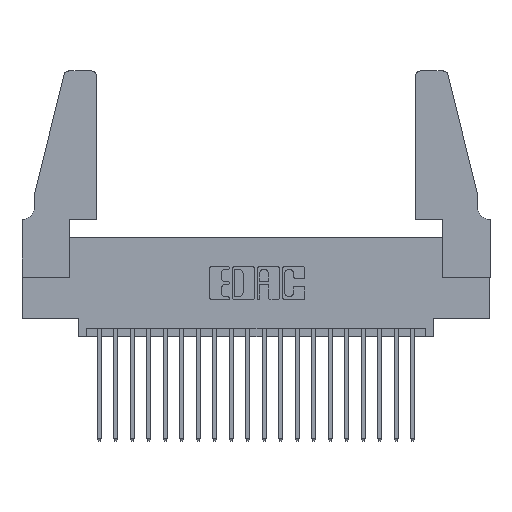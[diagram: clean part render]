
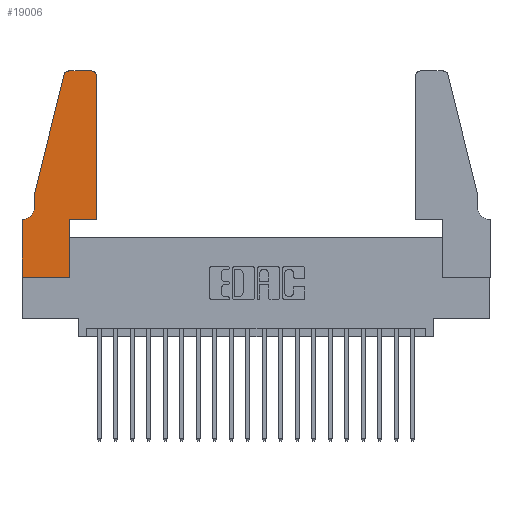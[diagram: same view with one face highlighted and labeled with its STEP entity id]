
A CAD part, top view. The second image highlights one B-rep face of the part: STEP entity #19006.
In plain terms, the highlighted planar face has unit normal (0, 0, 1).
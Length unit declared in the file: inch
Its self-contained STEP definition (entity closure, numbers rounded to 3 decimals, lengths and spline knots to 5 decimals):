
#118 = ORIENTED_EDGE ( 'NONE', *, *, #17093, .T. ) ;
#174 = LINE ( 'NONE', #9430, #17490 ) ;
#403 = CARTESIAN_POINT ( 'NONE',  ( 0.2865, 0., 0.37 ) ) ;
#721 = VERTEX_POINT ( 'NONE', #2761 ) ;
#1206 = ORIENTED_EDGE ( 'NONE', *, *, #18844, .T. ) ;
#1313 = VERTEX_POINT ( 'NONE', #9308 ) ;
#1337 = CARTESIAN_POINT ( 'NONE',  ( 0.0755, 0.42, 0.37 ) ) ;
#1368 = LINE ( 'NONE', #7653, #4801 ) ;
#1587 = EDGE_CURVE ( 'NONE', #721, #8507, #1368, .T. ) ;
#1672 = EDGE_CURVE ( 'NONE', #16099, #2057, #3743, .T. ) ;
#2003 = CARTESIAN_POINT ( 'NONE',  ( 0.0055, 0.35, 0.37 ) ) ;
#2057 = VERTEX_POINT ( 'NONE', #11794 ) ;
#2196 = DIRECTION ( 'NONE',  ( -1., 0., 0. ) ) ;
#2416 = LINE ( 'NONE', #7904, #14903 ) ;
#2524 = ORIENTED_EDGE ( 'NONE', *, *, #1587, .T. ) ;
#2761 = CARTESIAN_POINT ( 'NONE',  ( 0.0755, 0.5, 0.37 ) ) ;
#2979 = DIRECTION ( 'NONE',  ( 1., 0., 0. ) ) ;
#2988 = ORIENTED_EDGE ( 'NONE', *, *, #8471, .T. ) ;
#3020 = AXIS2_PLACEMENT_3D ( 'NONE', #13371, #3627, #14956 ) ;
#3223 = VECTOR ( 'NONE', #11730, 39.37008 ) ;
#3501 = VERTEX_POINT ( 'NONE', #4126 ) ;
#3627 = DIRECTION ( 'NONE',  ( 0., 0., -1. ) ) ;
#3743 = LINE ( 'NONE', #11330, #3223 ) ;
#3797 = CARTESIAN_POINT ( 'NONE',  ( 0., 0.35, 0.37 ) ) ;
#3916 = CARTESIAN_POINT ( 'NONE',  ( 0.2605, 1.25, 0.37 ) ) ;
#4104 = VERTEX_POINT ( 'NONE', #10342 ) ;
#4126 = CARTESIAN_POINT ( 'NONE',  ( 0.284, 1.25, 0.37 ) ) ;
#4167 = CIRCLE ( 'NONE', #3020, 0.07 ) ;
#4284 = CARTESIAN_POINT ( 'NONE',  ( 0., 0., 0.37 ) ) ;
#4291 = DIRECTION ( 'NONE',  ( 0., 0., 1. ) ) ;
#4454 = ORIENTED_EDGE ( 'NONE', *, *, #9202, .T. ) ;
#4553 = CARTESIAN_POINT ( 'NONE',  ( 0.0755, 0.35, 0.37 ) ) ;
#4801 = VECTOR ( 'NONE', #13757, 39.37008 ) ;
#5517 = EDGE_CURVE ( 'NONE', #1313, #721, #19964, .T. ) ;
#5523 = VECTOR ( 'NONE', #17160, 39.37008 ) ;
#6093 = CARTESIAN_POINT ( 'NONE',  ( 0.284, 1.22, 0.37 ) ) ;
#6197 = ORIENTED_EDGE ( 'NONE', *, *, #1672, .T. ) ;
#6291 = ORIENTED_EDGE ( 'NONE', *, *, #14960, .T. ) ;
#6374 = CARTESIAN_POINT ( 'NONE',  ( 0., 0.35, 0.37 ) ) ;
#7531 = VECTOR ( 'NONE', #17345, 39.37008 ) ;
#7577 = ORIENTED_EDGE ( 'NONE', *, *, #10851, .T. ) ;
#7653 = CARTESIAN_POINT ( 'NONE',  ( 0.0755, 0.5, 0.37 ) ) ;
#7717 = DIRECTION ( 'NONE',  ( 0., 1., 0. ) ) ;
#7752 = DIRECTION ( 'NONE',  ( 1., 0., 0. ) ) ;
#7781 = CIRCLE ( 'NONE', #16152, 0.03 ) ;
#7857 = CARTESIAN_POINT ( 'NONE',  ( 0.4505, 0.35, 0.37 ) ) ;
#7876 = LINE ( 'NONE', #3916, #11656 ) ;
#7904 = CARTESIAN_POINT ( 'NONE',  ( 0., 0., 0.37 ) ) ;
#8020 = DIRECTION ( 'NONE',  ( 1., 0., 0. ) ) ;
#8045 = LINE ( 'NONE', #4553, #7531 ) ;
#8194 = ORIENTED_EDGE ( 'NONE', *, *, #17088, .T. ) ;
#8471 = EDGE_CURVE ( 'NONE', #10983, #10226, #2416, .T. ) ;
#8507 = VERTEX_POINT ( 'NONE', #1337 ) ;
#8801 = CARTESIAN_POINT ( 'NONE',  ( 0., 0., 0.37 ) ) ;
#8849 = EDGE_CURVE ( 'NONE', #11678, #3501, #7876, .T. ) ;
#8924 = CARTESIAN_POINT ( 'NONE',  ( 0.4205, 1.25, 0.37 ) ) ;
#9202 = EDGE_CURVE ( 'NONE', #15530, #10983, #9892, .T. ) ;
#9308 = CARTESIAN_POINT ( 'NONE',  ( 0.25487, 1.22718, 0.37 ) ) ;
#9430 = CARTESIAN_POINT ( 'NONE',  ( 0.2865, 0.35, 0.37 ) ) ;
#9485 = DIRECTION ( 'NONE',  ( 1., 0., 0. ) ) ;
#9892 = LINE ( 'NONE', #4284, #5523 ) ;
#10226 = VERTEX_POINT ( 'NONE', #403 ) ;
#10281 = ORIENTED_EDGE ( 'NONE', *, *, #8849, .T. ) ;
#10342 = CARTESIAN_POINT ( 'NONE',  ( 0.2865, 0.35, 0.37 ) ) ;
#10851 = EDGE_CURVE ( 'NONE', #8507, #15477, #4167, .T. ) ;
#10983 = VERTEX_POINT ( 'NONE', #8801 ) ;
#11314 = AXIS2_PLACEMENT_3D ( 'NONE', #6093, #17316, #7752 ) ;
#11330 = CARTESIAN_POINT ( 'NONE',  ( 0.4505, 0.35, 0.37 ) ) ;
#11512 = AXIS2_PLACEMENT_3D ( 'NONE', #6374, #17588, #8020 ) ;
#11543 = EDGE_LOOP ( 'NONE', ( #10281, #6291, #12653, #2524, #7577, #8194, #4454, #2988, #20379, #118, #6197, #1206 ) ) ;
#11554 = VECTOR ( 'NONE', #16802, 39.37008 ) ;
#11656 = VECTOR ( 'NONE', #2196, 39.37008 ) ;
#11678 = VERTEX_POINT ( 'NONE', #8924 ) ;
#11730 = DIRECTION ( 'NONE',  ( 0., 1., 0. ) ) ;
#11794 = CARTESIAN_POINT ( 'NONE',  ( 0.4505, 1.22, 0.37 ) ) ;
#11829 = CARTESIAN_POINT ( 'NONE',  ( 0.4505, 0.35, 0.37 ) ) ;
#11891 = EDGE_CURVE ( 'NONE', #10226, #4104, #174, .T. ) ;
#12023 = CARTESIAN_POINT ( 'NONE',  ( 0.0755, 0.5, 0.37 ) ) ;
#12653 = ORIENTED_EDGE ( 'NONE', *, *, #5517, .T. ) ;
#12817 = PLANE ( 'NONE',  #11512 ) ;
#13371 = CARTESIAN_POINT ( 'NONE',  ( 0.0055, 0.42, 0.37 ) ) ;
#13757 = DIRECTION ( 'NONE',  ( 0., -1., 0. ) ) ;
#13994 = CARTESIAN_POINT ( 'NONE',  ( 0.4205, 1.22, 0.37 ) ) ;
#14903 = VECTOR ( 'NONE', #2979, 39.37008 ) ;
#14956 = DIRECTION ( 'NONE',  ( -1., 0., 0. ) ) ;
#14960 = EDGE_CURVE ( 'NONE', #3501, #1313, #17130, .T. ) ;
#15477 = VERTEX_POINT ( 'NONE', #2003 ) ;
#15530 = VERTEX_POINT ( 'NONE', #3797 ) ;
#15586 = DIRECTION ( 'NONE',  ( 1., 0., 0. ) ) ;
#16043 = LINE ( 'NONE', #7857, #19741 ) ;
#16099 = VERTEX_POINT ( 'NONE', #11829 ) ;
#16152 = AXIS2_PLACEMENT_3D ( 'NONE', #13994, #4291, #15586 ) ;
#16802 = DIRECTION ( 'NONE',  ( -0.239, -0.971, 0. ) ) ;
#16993 = FACE_OUTER_BOUND ( 'NONE', #11543, .T. ) ;
#17088 = EDGE_CURVE ( 'NONE', #15477, #15530, #8045, .T. ) ;
#17093 = EDGE_CURVE ( 'NONE', #4104, #16099, #16043, .T. ) ;
#17130 = CIRCLE ( 'NONE', #11314, 0.03 ) ;
#17160 = DIRECTION ( 'NONE',  ( 0., -1., 0. ) ) ;
#17316 = DIRECTION ( 'NONE',  ( 0., 0., 1. ) ) ;
#17345 = DIRECTION ( 'NONE',  ( -1., 0., 0. ) ) ;
#17490 = VECTOR ( 'NONE', #7717, 39.37008 ) ;
#17588 = DIRECTION ( 'NONE',  ( 0., 0., 1. ) ) ;
#18844 = EDGE_CURVE ( 'NONE', #2057, #11678, #7781, .T. ) ;
#19006 = ADVANCED_FACE ( 'NONE', ( #16993 ), #12817, .T. ) ;
#19741 = VECTOR ( 'NONE', #9485, 39.37008 ) ;
#19964 = LINE ( 'NONE', #12023, #11554 ) ;
#20379 = ORIENTED_EDGE ( 'NONE', *, *, #11891, .T. ) ;
